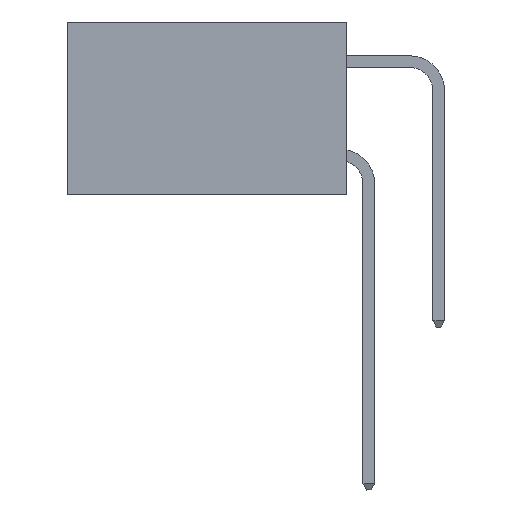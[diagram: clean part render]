
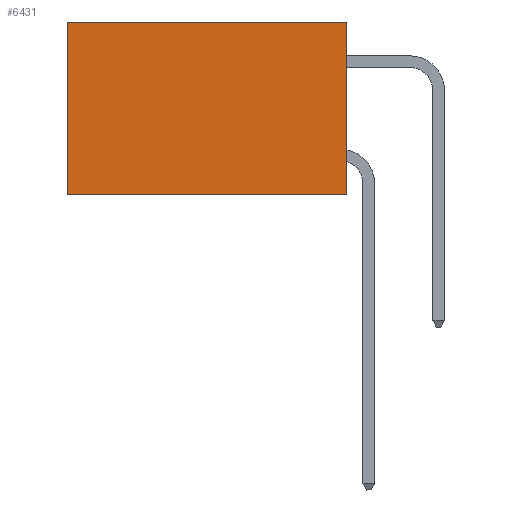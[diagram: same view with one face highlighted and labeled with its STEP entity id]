
A CAD part, left-side view. The second image highlights one B-rep face of the part: STEP entity #6431.
In plain terms, the highlighted planar face has unit normal (-1, 0, 0).
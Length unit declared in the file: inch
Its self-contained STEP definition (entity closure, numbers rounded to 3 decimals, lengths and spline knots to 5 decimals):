
#425 = CARTESIAN_POINT ( 'NONE',  ( 0.2875, 0.6, 0. ) ) ;
#804 = EDGE_CURVE ( 'NONE', #1580, #16933, #5971, .T. ) ;
#904 = CARTESIAN_POINT ( 'NONE',  ( 0.2875, 0., 0. ) ) ;
#1151 = ORIENTED_EDGE ( 'NONE', *, *, #26891, .T. ) ;
#1580 = VERTEX_POINT ( 'NONE', #904 ) ;
#1624 = DIRECTION ( 'NONE',  ( 0., 0., -1. ) ) ;
#1634 = DIRECTION ( 'NONE',  ( 0., 1., 0. ) ) ;
#2003 = CARTESIAN_POINT ( 'NONE',  ( 0.2875, 0., 0. ) ) ;
#3285 = CARTESIAN_POINT ( 'NONE',  ( 0.2875, 0.6, 0. ) ) ;
#3975 = VECTOR ( 'NONE', #15070, 39.37008 ) ;
#4444 = LINE ( 'NONE', #25228, #20287 ) ;
#5182 = CARTESIAN_POINT ( 'NONE',  ( 0.2875, 0., -0.37 ) ) ;
#5454 = DIRECTION ( 'NONE',  ( 0., 0., -1. ) ) ;
#5971 = LINE ( 'NONE', #23494, #11042 ) ;
#6086 = VECTOR ( 'NONE', #5454, 39.37008 ) ;
#6431 = ADVANCED_FACE ( 'NONE', ( #9066 ), #23225, .F. ) ;
#6773 = ORIENTED_EDGE ( 'NONE', *, *, #804, .F. ) ;
#8805 = EDGE_CURVE ( 'NONE', #25759, #21962, #23213, .T. ) ;
#9066 = FACE_OUTER_BOUND ( 'NONE', #15403, .T. ) ;
#10418 = DIRECTION ( 'NONE',  ( 1., 0., 0. ) ) ;
#10431 = LINE ( 'NONE', #2003, #3975 ) ;
#10901 = ORIENTED_EDGE ( 'NONE', *, *, #8805, .T. ) ;
#11042 = VECTOR ( 'NONE', #1624, 39.37008 ) ;
#12459 = CARTESIAN_POINT ( 'NONE',  ( 0.2875, 0., 0. ) ) ;
#15070 = DIRECTION ( 'NONE',  ( 0., 1., 0. ) ) ;
#15403 = EDGE_LOOP ( 'NONE', ( #10901, #15769, #6773, #1151 ) ) ;
#15769 = ORIENTED_EDGE ( 'NONE', *, *, #24351, .F. ) ;
#16933 = VERTEX_POINT ( 'NONE', #5182 ) ;
#19449 = CARTESIAN_POINT ( 'NONE',  ( 0.2875, 0.6, -0.37 ) ) ;
#20287 = VECTOR ( 'NONE', #1634, 39.37008 ) ;
#21962 = VERTEX_POINT ( 'NONE', #19449 ) ;
#23213 = LINE ( 'NONE', #3285, #6086 ) ;
#23225 = PLANE ( 'NONE',  #23828 ) ;
#23494 = CARTESIAN_POINT ( 'NONE',  ( 0.2875, 0., 0. ) ) ;
#23828 = AXIS2_PLACEMENT_3D ( 'NONE', #12459, #10418, #25334 ) ;
#24351 = EDGE_CURVE ( 'NONE', #16933, #21962, #4444, .T. ) ;
#25228 = CARTESIAN_POINT ( 'NONE',  ( 0.2875, 0., -0.37 ) ) ;
#25334 = DIRECTION ( 'NONE',  ( 0., 0., -1. ) ) ;
#25759 = VERTEX_POINT ( 'NONE', #425 ) ;
#26891 = EDGE_CURVE ( 'NONE', #1580, #25759, #10431, .T. ) ;
